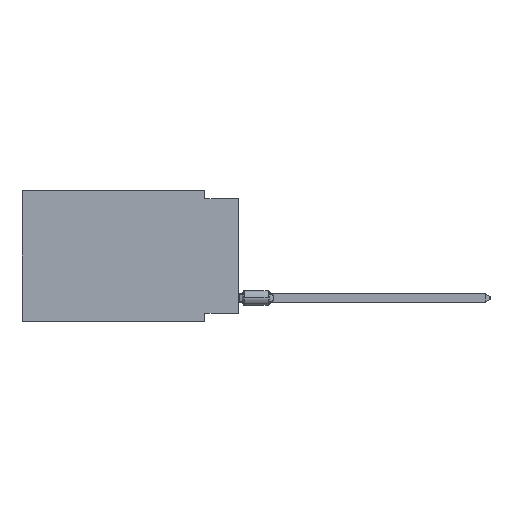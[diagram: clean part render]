
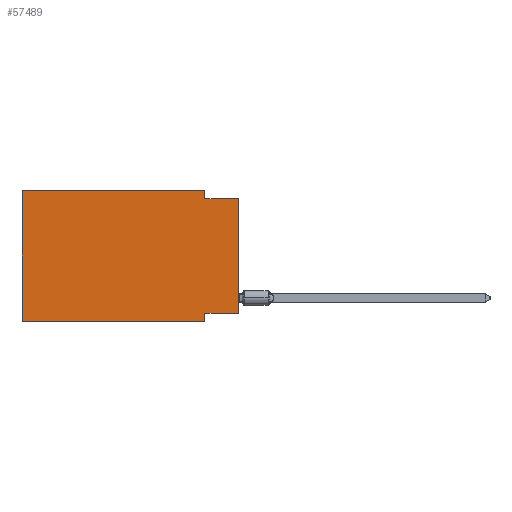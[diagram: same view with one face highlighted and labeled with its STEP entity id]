
A CAD part, left-side view. The second image highlights one B-rep face of the part: STEP entity #57489.
In plain terms, the highlighted planar face has unit normal (-1, 0, 0).
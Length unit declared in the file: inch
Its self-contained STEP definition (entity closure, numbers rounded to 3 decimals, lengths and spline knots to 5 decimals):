
#1100 = ORIENTED_EDGE ( 'NONE', *, *, #54262, .F. ) ;
#1487 = LINE ( 'NONE', #45490, #57145 ) ;
#1751 = CARTESIAN_POINT ( 'NONE',  ( 0., 0.1, -0.025 ) ) ;
#3443 = CARTESIAN_POINT ( 'NONE',  ( 0., 0.645, 0. ) ) ;
#3525 = CARTESIAN_POINT ( 'NONE',  ( 0., 0.645, 0. ) ) ;
#5160 = VERTEX_POINT ( 'NONE', #52255 ) ;
#5176 = DIRECTION ( 'NONE',  ( 0., -1., 0. ) ) ;
#6269 = DIRECTION ( 'NONE',  ( 1., 0., 0. ) ) ;
#7663 = ORIENTED_EDGE ( 'NONE', *, *, #30423, .T. ) ;
#8425 = EDGE_CURVE ( 'NONE', #5160, #75558, #49745, .T. ) ;
#8914 = VECTOR ( 'NONE', #12281, 39.37008 ) ;
#9632 = DIRECTION ( 'NONE',  ( 0., 1., 0. ) ) ;
#11450 = ORIENTED_EDGE ( 'NONE', *, *, #8425, .F. ) ;
#11535 = CARTESIAN_POINT ( 'NONE',  ( 0., 0.645, 0. ) ) ;
#12281 = DIRECTION ( 'NONE',  ( 0., -1., 0. ) ) ;
#15691 = LINE ( 'NONE', #53668, #50493 ) ;
#16054 = LINE ( 'NONE', #3525, #8914 ) ;
#17382 = VECTOR ( 'NONE', #74409, 39.37008 ) ;
#19755 = EDGE_CURVE ( 'NONE', #60940, #41729, #51369, .T. ) ;
#21632 = LINE ( 'NONE', #3443, #70452 ) ;
#23491 = VERTEX_POINT ( 'NONE', #44470 ) ;
#24651 = CARTESIAN_POINT ( 'NONE',  ( 0., 0., -0.365 ) ) ;
#24962 = VECTOR ( 'NONE', #49795, 39.37008 ) ;
#26906 = DIRECTION ( 'NONE',  ( 0., 0., -1. ) ) ;
#27740 = EDGE_CURVE ( 'NONE', #76513, #5160, #15691, .T. ) ;
#30423 = EDGE_CURVE ( 'NONE', #66299, #75558, #44319, .T. ) ;
#31929 = VECTOR ( 'NONE', #5176, 39.37008 ) ;
#32219 = DIRECTION ( 'NONE',  ( 0., -1., 0. ) ) ;
#32688 = ORIENTED_EDGE ( 'NONE', *, *, #54463, .T. ) ;
#35789 = DIRECTION ( 'NONE',  ( 0., 0., -1. ) ) ;
#36812 = CARTESIAN_POINT ( 'NONE',  ( 0., 0.1, -0.39 ) ) ;
#36933 = EDGE_CURVE ( 'NONE', #23491, #50579, #16054, .T. ) ;
#36978 = FACE_OUTER_BOUND ( 'NONE', #62715, .T. ) ;
#41729 = VERTEX_POINT ( 'NONE', #45353 ) ;
#43575 = ORIENTED_EDGE ( 'NONE', *, *, #36933, .F. ) ;
#44319 = LINE ( 'NONE', #63340, #48244 ) ;
#44470 = CARTESIAN_POINT ( 'NONE',  ( 0., 0.645, 0. ) ) ;
#44503 = LINE ( 'NONE', #67988, #24962 ) ;
#44655 = ORIENTED_EDGE ( 'NONE', *, *, #19755, .F. ) ;
#45353 = CARTESIAN_POINT ( 'NONE',  ( 0., 0., -0.025 ) ) ;
#45490 = CARTESIAN_POINT ( 'NONE',  ( 0., 0.1, 0. ) ) ;
#46890 = ORIENTED_EDGE ( 'NONE', *, *, #73108, .F. ) ;
#47089 = CARTESIAN_POINT ( 'NONE',  ( 0., 0.1, -0.39 ) ) ;
#48244 = VECTOR ( 'NONE', #32219, 39.37008 ) ;
#49745 = LINE ( 'NONE', #36812, #17382 ) ;
#49795 = DIRECTION ( 'NONE',  ( 0., 0., 1. ) ) ;
#50493 = VECTOR ( 'NONE', #9632, 39.37008 ) ;
#50579 = VERTEX_POINT ( 'NONE', #70293 ) ;
#51369 = LINE ( 'NONE', #76029, #31929 ) ;
#52255 = CARTESIAN_POINT ( 'NONE',  ( 0., 0.1, -0.365 ) ) ;
#53668 = CARTESIAN_POINT ( 'NONE',  ( 0., 0., -0.365 ) ) ;
#54262 = EDGE_CURVE ( 'NONE', #50579, #60940, #1487, .T. ) ;
#54463 = EDGE_CURVE ( 'NONE', #76513, #41729, #44503, .T. ) ;
#57145 = VECTOR ( 'NONE', #26906, 39.37008 ) ;
#57489 = ADVANCED_FACE ( 'NONE', ( #36978 ), #61655, .F. ) ;
#60723 = CARTESIAN_POINT ( 'NONE',  ( 0., 0.645, -0.39 ) ) ;
#60940 = VERTEX_POINT ( 'NONE', #1751 ) ;
#61250 = AXIS2_PLACEMENT_3D ( 'NONE', #11535, #6269, #35789 ) ;
#61655 = PLANE ( 'NONE',  #61250 ) ;
#62715 = EDGE_LOOP ( 'NONE', ( #32688, #44655, #1100, #43575, #46890, #7663, #11450, #77286 ) ) ;
#63340 = CARTESIAN_POINT ( 'NONE',  ( 0., 0.645, -0.39 ) ) ;
#66299 = VERTEX_POINT ( 'NONE', #60723 ) ;
#67988 = CARTESIAN_POINT ( 'NONE',  ( 0., 0., 0. ) ) ;
#70293 = CARTESIAN_POINT ( 'NONE',  ( 0., 0.1, 0. ) ) ;
#70452 = VECTOR ( 'NONE', #70925, 39.37008 ) ;
#70925 = DIRECTION ( 'NONE',  ( 0., 0., 1. ) ) ;
#73108 = EDGE_CURVE ( 'NONE', #66299, #23491, #21632, .T. ) ;
#74409 = DIRECTION ( 'NONE',  ( 0., 0., -1. ) ) ;
#75558 = VERTEX_POINT ( 'NONE', #47089 ) ;
#76029 = CARTESIAN_POINT ( 'NONE',  ( 0., 0., -0.025 ) ) ;
#76513 = VERTEX_POINT ( 'NONE', #24651 ) ;
#77286 = ORIENTED_EDGE ( 'NONE', *, *, #27740, .F. ) ;
